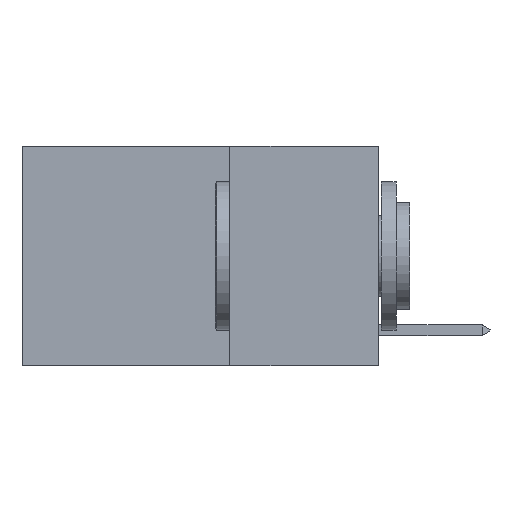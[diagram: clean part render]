
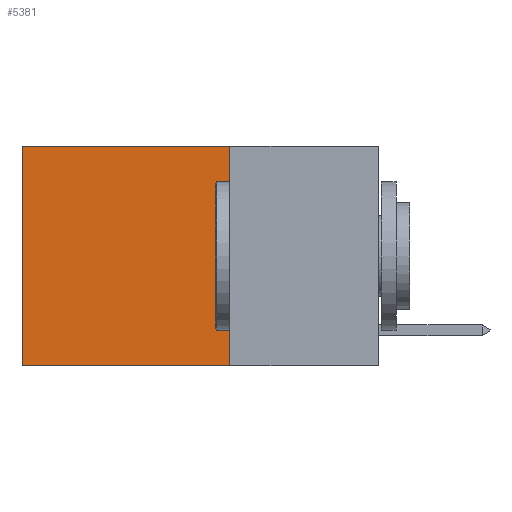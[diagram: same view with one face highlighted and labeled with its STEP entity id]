
A CAD part, left-side view. The second image highlights one B-rep face of the part: STEP entity #5381.
In plain terms, the highlighted planar face has unit normal (-1, 0, 0).
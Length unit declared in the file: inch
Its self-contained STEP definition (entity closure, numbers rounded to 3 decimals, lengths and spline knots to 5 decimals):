
#372 = FACE_OUTER_BOUND ( 'NONE', #813, .T. ) ;
#458 = DIRECTION ( 'NONE',  ( 0., 0., -1. ) ) ;
#813 = EDGE_LOOP ( 'NONE', ( #1140, #4329, #3851, #11789 ) ) ;
#843 = CARTESIAN_POINT ( 'NONE',  ( 0.2625, 0.6, 0. ) ) ;
#1140 = ORIENTED_EDGE ( 'NONE', *, *, #2499, .T. ) ;
#1675 = VERTEX_POINT ( 'NONE', #17379 ) ;
#2071 = VECTOR ( 'NONE', #6830, 39.37008 ) ;
#2499 = EDGE_CURVE ( 'NONE', #3570, #4128, #13936, .T. ) ;
#2531 = LINE ( 'NONE', #3961, #2071 ) ;
#2996 = VECTOR ( 'NONE', #458, 39.37008 ) ;
#3064 = VECTOR ( 'NONE', #11327, 39.37008 ) ;
#3376 = EDGE_CURVE ( 'NONE', #1675, #3570, #16885, .T. ) ;
#3570 = VERTEX_POINT ( 'NONE', #8842 ) ;
#3851 = ORIENTED_EDGE ( 'NONE', *, *, #4757, .F. ) ;
#3961 = CARTESIAN_POINT ( 'NONE',  ( 0.2625, 0.25, 0. ) ) ;
#4128 = VERTEX_POINT ( 'NONE', #15539 ) ;
#4139 = CARTESIAN_POINT ( 'NONE',  ( 0.2625, 0.25, 0. ) ) ;
#4202 = DIRECTION ( 'NONE',  ( 1., 0., 0. ) ) ;
#4329 = ORIENTED_EDGE ( 'NONE', *, *, #5787, .F. ) ;
#4757 = EDGE_CURVE ( 'NONE', #1675, #4960, #2531, .T. ) ;
#4960 = VERTEX_POINT ( 'NONE', #15268 ) ;
#5381 = ADVANCED_FACE ( 'NONE', ( #372 ), #11146, .F. ) ;
#5787 = EDGE_CURVE ( 'NONE', #4960, #4128, #12288, .T. ) ;
#6830 = DIRECTION ( 'NONE',  ( 0., 0., -1. ) ) ;
#8271 = VECTOR ( 'NONE', #13725, 39.37008 ) ;
#8842 = CARTESIAN_POINT ( 'NONE',  ( 0.2625, 0.6, 0. ) ) ;
#11146 = PLANE ( 'NONE',  #11455 ) ;
#11288 = CARTESIAN_POINT ( 'NONE',  ( 0.2625, 0.25, 0. ) ) ;
#11327 = DIRECTION ( 'NONE',  ( 0., 1., 0. ) ) ;
#11455 = AXIS2_PLACEMENT_3D ( 'NONE', #4139, #4202, #13739 ) ;
#11789 = ORIENTED_EDGE ( 'NONE', *, *, #3376, .T. ) ;
#12288 = LINE ( 'NONE', #12449, #8271 ) ;
#12449 = CARTESIAN_POINT ( 'NONE',  ( 0.2625, 0.25, -0.37 ) ) ;
#13725 = DIRECTION ( 'NONE',  ( 0., 1., 0. ) ) ;
#13739 = DIRECTION ( 'NONE',  ( 0., 0., -1. ) ) ;
#13936 = LINE ( 'NONE', #843, #2996 ) ;
#15268 = CARTESIAN_POINT ( 'NONE',  ( 0.2625, 0.25, -0.37 ) ) ;
#15539 = CARTESIAN_POINT ( 'NONE',  ( 0.2625, 0.6, -0.37 ) ) ;
#16885 = LINE ( 'NONE', #11288, #3064 ) ;
#17379 = CARTESIAN_POINT ( 'NONE',  ( 0.2625, 0.25, 0. ) ) ;
